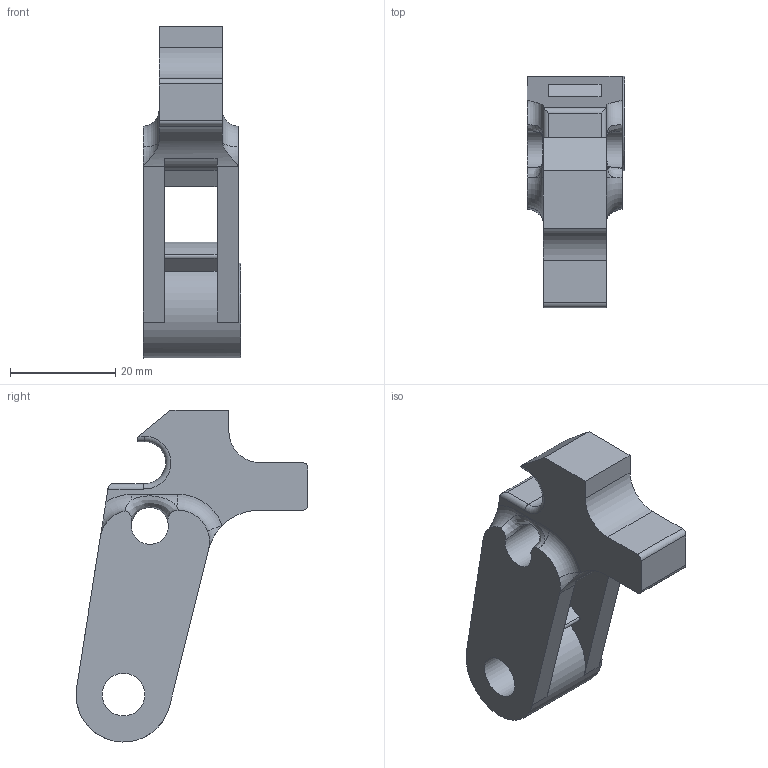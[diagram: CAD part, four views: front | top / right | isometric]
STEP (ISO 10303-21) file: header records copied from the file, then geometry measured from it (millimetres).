
FILE_DESCRIPTION((''),'2;1');
FILE_NAME('PM422Hammer2.stp','2015-08-22T19:02:44',('JamesRPatrick'),(''),'Autodesk Inventor 2012','Autodesk Inventor 2012','');
FILE_SCHEMA(('AUTOMOTIVE_DESIGN { 1 0 10303 214 1 1 1 1 }'));
Length unit declared in the file: millimetre
Products named in the file (1): PM422Hammer2
Bounding box: 18.5 x 44 x 63 mm (x, y, z)
Volume: 15821.1 mm3; surface area: 6808.4 mm2
Topology: 1 solids, 1 shells, 52 faces, 149 edges, 96 vertices
Faces by surface type: plane 21, cylinder 21, torus 8, bspline 2
Full cylindrical faces by diameter (mm): 7 x1, 8.1 x1, 18 x1
Entity records: 2151 total; most frequent: CARTESIAN_POINT 764, ORIENTED_EDGE 290, DIRECTION 286, EDGE_CURVE 145, AXIS2_PLACEMENT_3D 110, VERTEX_POINT 95, VECTOR 66, LINE 66
